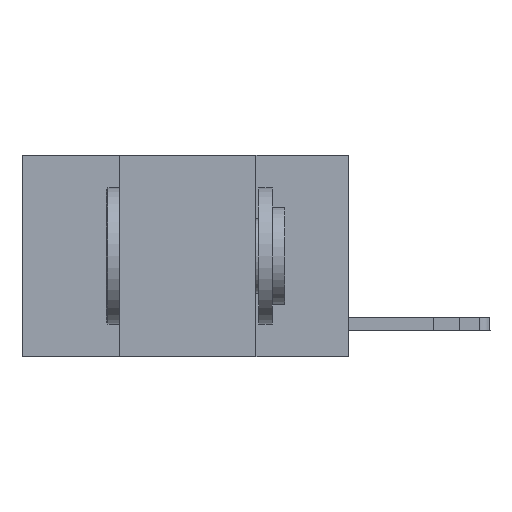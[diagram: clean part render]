
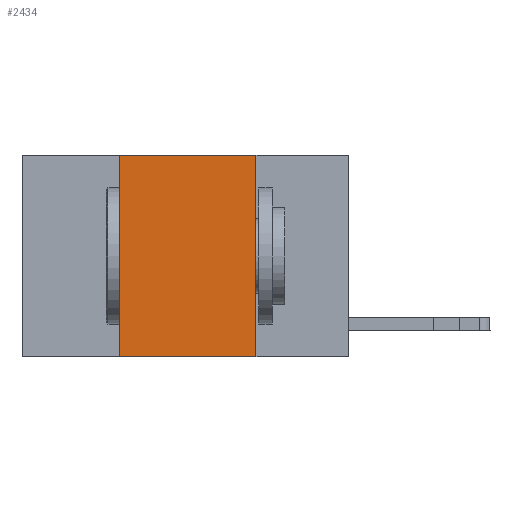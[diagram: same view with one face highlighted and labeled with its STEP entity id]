
A CAD part, left-side view. The second image highlights one B-rep face of the part: STEP entity #2434.
In plain terms, the highlighted planar face has unit normal (-1, 0, 0).
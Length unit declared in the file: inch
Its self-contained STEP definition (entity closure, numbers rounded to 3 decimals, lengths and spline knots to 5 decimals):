
#19 = CARTESIAN_POINT ( 'NONE',  ( 0., 0.17, -0.37 ) ) ;
#1511 = ORIENTED_EDGE ( 'NONE', *, *, #12728, .F. ) ;
#2434 = ADVANCED_FACE ( 'NONE', ( #14711 ), #2890, .F. ) ;
#2791 = LINE ( 'NONE', #12792, #17298 ) ;
#2890 = PLANE ( 'NONE',  #3705 ) ;
#3304 = DIRECTION ( 'NONE',  ( 0., -1., 0. ) ) ;
#3705 = AXIS2_PLACEMENT_3D ( 'NONE', #13285, #20951, #9046 ) ;
#4940 = CARTESIAN_POINT ( 'NONE',  ( 0., 0.17, 0. ) ) ;
#6737 = EDGE_CURVE ( 'NONE', #14797, #22856, #19196, .T. ) ;
#6891 = LINE ( 'NONE', #4940, #15622 ) ;
#8518 = ORIENTED_EDGE ( 'NONE', *, *, #6737, .T. ) ;
#9046 = DIRECTION ( 'NONE',  ( 0., 0., -1. ) ) ;
#9745 = LINE ( 'NONE', #17645, #10554 ) ;
#10554 = VECTOR ( 'NONE', #21697, 39.37008 ) ;
#11850 = CARTESIAN_POINT ( 'NONE',  ( 0., 0.17, 0. ) ) ;
#12728 = EDGE_CURVE ( 'NONE', #17720, #16177, #2791, .T. ) ;
#12792 = CARTESIAN_POINT ( 'NONE',  ( 0., 0.6, 0. ) ) ;
#13285 = CARTESIAN_POINT ( 'NONE',  ( 0., 0.6, 0. ) ) ;
#13895 = VECTOR ( 'NONE', #25592, 39.37008 ) ;
#14711 = FACE_OUTER_BOUND ( 'NONE', #17166, .T. ) ;
#14797 = VERTEX_POINT ( 'NONE', #24953 ) ;
#15622 = VECTOR ( 'NONE', #16191, 39.37008 ) ;
#16177 = VERTEX_POINT ( 'NONE', #11850 ) ;
#16191 = DIRECTION ( 'NONE',  ( 0., 0., -1. ) ) ;
#16722 = EDGE_CURVE ( 'NONE', #14797, #17720, #9745, .T. ) ;
#17166 = EDGE_LOOP ( 'NONE', ( #25371, #1511, #24495, #8518 ) ) ;
#17298 = VECTOR ( 'NONE', #3304, 39.37008 ) ;
#17645 = CARTESIAN_POINT ( 'NONE',  ( 0., 0.42, 0. ) ) ;
#17720 = VERTEX_POINT ( 'NONE', #22369 ) ;
#18082 = EDGE_CURVE ( 'NONE', #16177, #22856, #6891, .T. ) ;
#19196 = LINE ( 'NONE', #21145, #13895 ) ;
#20951 = DIRECTION ( 'NONE',  ( 1., 0., 0. ) ) ;
#21145 = CARTESIAN_POINT ( 'NONE',  ( 0., 0.6, -0.37 ) ) ;
#21697 = DIRECTION ( 'NONE',  ( 0., 0., 1. ) ) ;
#22369 = CARTESIAN_POINT ( 'NONE',  ( 0., 0.42, 0. ) ) ;
#22856 = VERTEX_POINT ( 'NONE', #19 ) ;
#24495 = ORIENTED_EDGE ( 'NONE', *, *, #16722, .F. ) ;
#24953 = CARTESIAN_POINT ( 'NONE',  ( 0., 0.42, -0.37 ) ) ;
#25371 = ORIENTED_EDGE ( 'NONE', *, *, #18082, .F. ) ;
#25592 = DIRECTION ( 'NONE',  ( 0., -1., 0. ) ) ;
